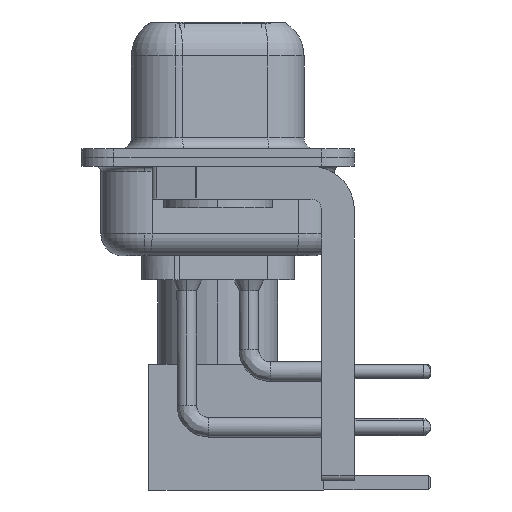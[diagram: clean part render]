
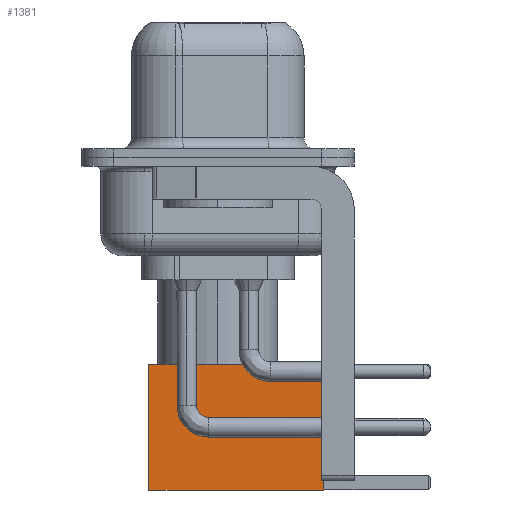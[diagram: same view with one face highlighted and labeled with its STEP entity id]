
A CAD part, left-side view. The second image highlights one B-rep face of the part: STEP entity #1381.
In plain terms, the highlighted face is planar.
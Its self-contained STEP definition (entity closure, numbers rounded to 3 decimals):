
#1381 = ADVANCED_FACE ( 'NONE', ( #12491 ), #19584, .T. ) ;
#1924 = DIRECTION ( 'NONE',  ( 0., 0., -1. ) ) ;
#3443 = VERTEX_POINT ( 'NONE', #17761 ) ;
#4182 = ORIENTED_EDGE ( 'NONE', *, *, #18160, .T. ) ;
#4257 = CARTESIAN_POINT ( 'NONE',  ( 2.875, 2.875, 0. ) ) ;
#4278 = VERTEX_POINT ( 'NONE', #4257 ) ;
#4812 = DIRECTION ( 'NONE',  ( 0., 1., 0. ) ) ;
#5007 = VECTOR ( 'NONE', #12669, 1000. ) ;
#5792 = VECTOR ( 'NONE', #18403, 1000. ) ;
#6483 = CARTESIAN_POINT ( 'NONE',  ( 2.875, 2.875, 0. ) ) ;
#6569 = CARTESIAN_POINT ( 'NONE',  ( 0., 2.875, 8. ) ) ;
#7474 = LINE ( 'NONE', #11066, #5792 ) ;
#7696 = DIRECTION ( 'NONE',  ( 0., 0., -1. ) ) ;
#8784 = AXIS2_PLACEMENT_3D ( 'NONE', #6483, #4812, #17784 ) ;
#9238 = LINE ( 'NONE', #20174, #19063 ) ;
#9590 = CARTESIAN_POINT ( 'NONE',  ( -2.875, 2.875, 8. ) ) ;
#9980 = CARTESIAN_POINT ( 'NONE',  ( 2.875, 2.875, 8. ) ) ;
#11066 = CARTESIAN_POINT ( 'NONE',  ( 0., 2.875, 0. ) ) ;
#12337 = ORIENTED_EDGE ( 'NONE', *, *, #15247, .F. ) ;
#12491 = FACE_OUTER_BOUND ( 'NONE', #18234, .T. ) ;
#12669 = DIRECTION ( 'NONE',  ( -1., 0., 0. ) ) ;
#13405 = ORIENTED_EDGE ( 'NONE', *, *, #16494, .F. ) ;
#13444 = CARTESIAN_POINT ( 'NONE',  ( 2.875, 2.875, 0. ) ) ;
#15247 = EDGE_CURVE ( 'NONE', #17719, #16669, #16165, .T. ) ;
#15881 = EDGE_CURVE ( 'NONE', #4278, #3443, #7474, .T. ) ;
#16165 = LINE ( 'NONE', #6569, #5007 ) ;
#16494 = EDGE_CURVE ( 'NONE', #16669, #3443, #9238, .T. ) ;
#16669 = VERTEX_POINT ( 'NONE', #9590 ) ;
#17044 = LINE ( 'NONE', #13444, #19912 ) ;
#17719 = VERTEX_POINT ( 'NONE', #9980 ) ;
#17761 = CARTESIAN_POINT ( 'NONE',  ( -2.875, 2.875, 0. ) ) ;
#17784 = DIRECTION ( 'NONE',  ( 0., 0., 1. ) ) ;
#18160 = EDGE_CURVE ( 'NONE', #17719, #4278, #17044, .T. ) ;
#18234 = EDGE_LOOP ( 'NONE', ( #4182, #20163, #13405, #12337 ) ) ;
#18403 = DIRECTION ( 'NONE',  ( -1., 0., 0. ) ) ;
#19063 = VECTOR ( 'NONE', #1924, 1000. ) ;
#19584 = PLANE ( 'NONE',  #8784 ) ;
#19912 = VECTOR ( 'NONE', #7696, 1000. ) ;
#20163 = ORIENTED_EDGE ( 'NONE', *, *, #15881, .T. ) ;
#20174 = CARTESIAN_POINT ( 'NONE',  ( -2.875, 2.875, 0. ) ) ;
